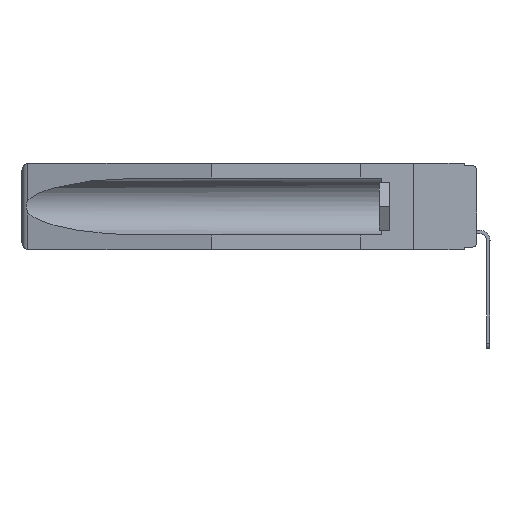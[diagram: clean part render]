
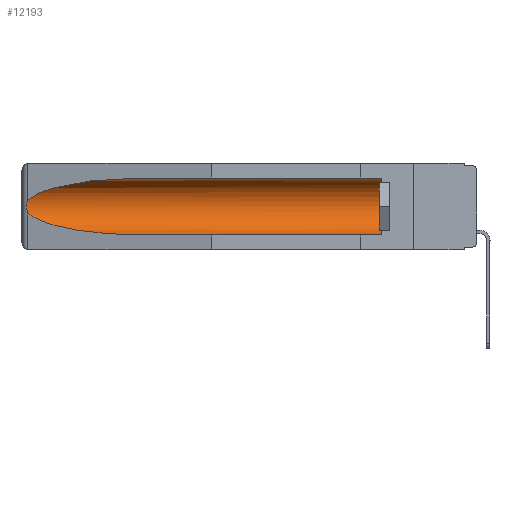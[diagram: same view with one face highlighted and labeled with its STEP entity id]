
A CAD part, left-side view. The second image highlights one B-rep face of the part: STEP entity #12193.
In plain terms, the highlighted cylindrical face has radius 2.857 mm (diameter 5.715 mm), a partial arc.
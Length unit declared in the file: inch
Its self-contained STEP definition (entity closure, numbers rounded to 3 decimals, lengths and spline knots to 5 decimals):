
#26 = ORIENTED_EDGE ( 'NONE', *, *, #6218, .T. ) ;
#45 = CARTESIAN_POINT ( 'NONE',  ( 0.26537, 1.52718, -0.14972 ) ) ;
#938 = LINE ( 'NONE', #10821, #9285 ) ;
#1819 = AXIS2_PLACEMENT_3D ( 'NONE', #20668, #18638, #21039 ) ;
#2768 = CARTESIAN_POINT ( 'NONE',  ( 0.155, 0.126, -0.059 ) ) ;
#2812 = EDGE_LOOP ( 'NONE', ( #19664, #26, #21134, #14708, #15123, #14943 ) ) ;
#3387 = DIRECTION ( 'NONE',  ( 0., -1., 0. ) ) ;
#3576 = DIRECTION ( 'NONE',  ( 0., 1., 0. ) ) ;
#4093 = CARTESIAN_POINT ( 'NONE',  ( 0.26654, 1.53092, -0.15636 ) ) ;
#5320 = CARTESIAN_POINT ( 'NONE',  ( 0.155, 0.126, -0.1715 ) ) ;
#5361 = VERTEX_POINT ( 'NONE', #45 ) ;
#5901 = CARTESIAN_POINT ( 'NONE',  ( 0.26537, 1.52718, -0.14972 ) ) ;
#5998 = CARTESIAN_POINT ( 'NONE',  ( 0.26537, 1.52718, -0.19328 ) ) ;
#6021 = CARTESIAN_POINT ( 'NONE',  ( 0.155, 1.07973, -0.284 ) ) ;
#6218 = EDGE_CURVE ( 'NONE', #5361, #22373, #10843, .T. ) ;
#6272 = CARTESIAN_POINT ( 'NONE',  ( 0.2673, 1.53269, -0.17917 ) ) ;
#6475 = CARTESIAN_POINT ( 'NONE',  ( 0.21114, 1.30732, -0.284 ) ) ;
#7359 = FACE_OUTER_BOUND ( 'NONE', #2812, .T. ) ;
#8471 = CARTESIAN_POINT ( 'NONE',  ( 0.155, 0.126, -0.284 ) ) ;
#9208 = CARTESIAN_POINT ( 'NONE',  ( 0.21114, 1.30732, -0.059 ) ) ;
#9285 = VECTOR ( 'NONE', #12373, 39.37008 ) ;
#9870 = CARTESIAN_POINT ( 'NONE',  ( 0.26537, 1.52718, -0.19328 ) ) ;
#9993 = CARTESIAN_POINT ( 'NONE',  ( 0.2675, 1.53308, -0.16763 ) ) ;
#10586 = VERTEX_POINT ( 'NONE', #11591 ) ;
#10821 = CARTESIAN_POINT ( 'NONE',  ( 0.155, -0.30754, -0.059 ) ) ;
#10843 = B_SPLINE_CURVE_WITH_KNOTS ( 'NONE', 3,
 ( #5901, #15998, #4093, #17682, #9993, #15870, #6272, #23329, #13591, #9870 ),
 .UNSPECIFIED., .F., .F.,
 ( 4, 2, 2, 2, 4 ),
 ( 0., 0.00029, 0.00058, 0.00087, 0.00117 ),
 .UNSPECIFIED. ) ;
#10896 = VECTOR ( 'NONE', #3576, 39.37008 ) ;
#11265 = EDGE_CURVE ( 'NONE', #10586, #5361, #18596, .T. ) ;
#11591 = CARTESIAN_POINT ( 'NONE',  ( 0.155, 1.07973, -0.059 ) ) ;
#12193 = ADVANCED_FACE ( 'NONE', ( #7359 ), #22978, .F. ) ;
#12373 = DIRECTION ( 'NONE',  ( 0., 1., 0. ) ) ;
#13147 = EDGE_CURVE ( 'NONE', #18567, #17432, #14042, .T. ) ;
#13209 =( BOUNDED_CURVE ( )  B_SPLINE_CURVE ( 3, ( #22459, #24036, #6475, #22081 ),
 .UNSPECIFIED., .F., .T. ) 
 B_SPLINE_CURVE_WITH_KNOTS ( ( 4, 4 ),
 ( 0.1948, 1.5708 ),
 .UNSPECIFIED. ) 
 CURVE ( )  GEOMETRIC_REPRESENTATION_ITEM ( )  RATIONAL_B_SPLINE_CURVE ( ( 1., 0.848, 0.848, 1. ) ) 
 REPRESENTATION_ITEM ( '' )  );
#13211 = EDGE_CURVE ( 'NONE', #20917, #10586, #938, .T. ) ;
#13281 = EDGE_CURVE ( 'NONE', #22373, #17432, #13209, .T. ) ;
#13465 = EDGE_CURVE ( 'NONE', #18567, #20917, #22039, .T. ) ;
#13591 = CARTESIAN_POINT ( 'NONE',  ( 0.26597, 1.5296, -0.19026 ) ) ;
#14042 = LINE ( 'NONE', #21110, #10896 ) ;
#14708 = ORIENTED_EDGE ( 'NONE', *, *, #13147, .F. ) ;
#14943 = ORIENTED_EDGE ( 'NONE', *, *, #13211, .T. ) ;
#15123 = ORIENTED_EDGE ( 'NONE', *, *, #13465, .T. ) ;
#15870 = CARTESIAN_POINT ( 'NONE',  ( 0.2675, 1.53308, -0.17534 ) ) ;
#15998 = CARTESIAN_POINT ( 'NONE',  ( 0.26597, 1.52961, -0.15275 ) ) ;
#17044 = CARTESIAN_POINT ( 'NONE',  ( 0.25451, 1.48313, -0.09465 ) ) ;
#17432 = VERTEX_POINT ( 'NONE', #6021 ) ;
#17682 = CARTESIAN_POINT ( 'NONE',  ( 0.2673, 1.5327, -0.16383 ) ) ;
#18567 = VERTEX_POINT ( 'NONE', #8471 ) ;
#18596 =( BOUNDED_CURVE ( )  B_SPLINE_CURVE ( 3, ( #19201, #9208, #17044, #18955 ),
 .UNSPECIFIED., .F., .F. ) 
 B_SPLINE_CURVE_WITH_KNOTS ( ( 4, 4 ),
 ( 4.71239, 6.08839 ),
 .UNSPECIFIED. ) 
 CURVE ( )  GEOMETRIC_REPRESENTATION_ITEM ( )  RATIONAL_B_SPLINE_CURVE ( ( 1., 0.848, 0.848, 1. ) ) 
 REPRESENTATION_ITEM ( '' )  );
#18638 = DIRECTION ( 'NONE',  ( 0., 1., 0. ) ) ;
#18955 = CARTESIAN_POINT ( 'NONE',  ( 0.26537, 1.52718, -0.14972 ) ) ;
#19201 = CARTESIAN_POINT ( 'NONE',  ( 0.155, 1.07973, -0.059 ) ) ;
#19664 = ORIENTED_EDGE ( 'NONE', *, *, #11265, .T. ) ;
#20668 = CARTESIAN_POINT ( 'NONE',  ( 0.155, -0.30754, -0.1715 ) ) ;
#20818 = AXIS2_PLACEMENT_3D ( 'NONE', #5320, #3387, #22722 ) ;
#20917 = VERTEX_POINT ( 'NONE', #2768 ) ;
#21039 = DIRECTION ( 'NONE',  ( 0., 0., 1. ) ) ;
#21110 = CARTESIAN_POINT ( 'NONE',  ( 0.155, -0.30754, -0.284 ) ) ;
#21134 = ORIENTED_EDGE ( 'NONE', *, *, #13281, .T. ) ;
#22039 = CIRCLE ( 'NONE', #20818, 0.1125 ) ;
#22081 = CARTESIAN_POINT ( 'NONE',  ( 0.155, 1.07973, -0.284 ) ) ;
#22373 = VERTEX_POINT ( 'NONE', #5998 ) ;
#22459 = CARTESIAN_POINT ( 'NONE',  ( 0.26537, 1.52718, -0.19328 ) ) ;
#22722 = DIRECTION ( 'NONE',  ( 0., 0., 1. ) ) ;
#22978 = CYLINDRICAL_SURFACE ( 'NONE', #1819, 0.1125 ) ;
#23329 = CARTESIAN_POINT ( 'NONE',  ( 0.26655, 1.53094, -0.18657 ) ) ;
#24036 = CARTESIAN_POINT ( 'NONE',  ( 0.25451, 1.48313, -0.24835 ) ) ;
